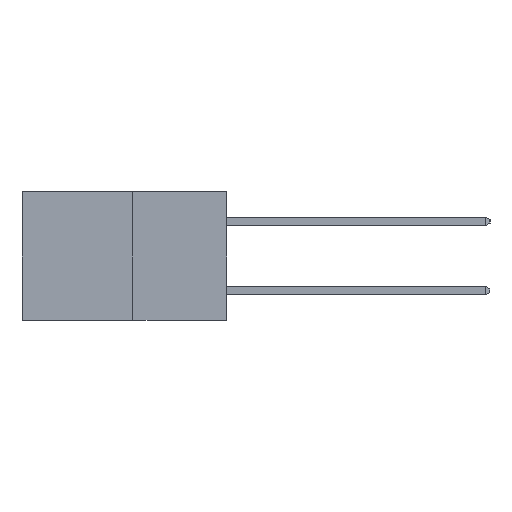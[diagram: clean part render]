
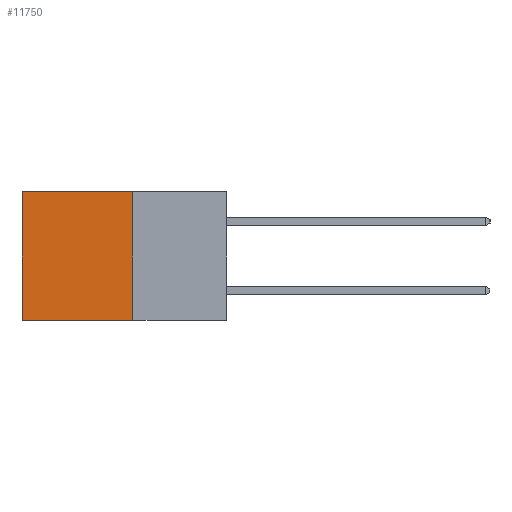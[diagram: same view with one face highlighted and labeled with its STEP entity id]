
A CAD part, left-side view. The second image highlights one B-rep face of the part: STEP entity #11750.
In plain terms, the highlighted planar face has unit normal (-1, 0, 0).
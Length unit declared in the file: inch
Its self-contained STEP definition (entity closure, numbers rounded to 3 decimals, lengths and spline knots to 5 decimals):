
#49 = ORIENTED_EDGE ( 'NONE', *, *, #5990, .T. ) ;
#1673 = LINE ( 'NONE', #11456, #5727 ) ;
#2010 = VERTEX_POINT ( 'NONE', #3660 ) ;
#2191 = DIRECTION ( 'NONE',  ( 0., 0., -1. ) ) ;
#3178 = EDGE_CURVE ( 'NONE', #15735, #7083, #20389, .T. ) ;
#3660 = CARTESIAN_POINT ( 'NONE',  ( 0.277, 0.27, 0. ) ) ;
#5144 = VECTOR ( 'NONE', #19757, 39.37008 ) ;
#5694 = LINE ( 'NONE', #19923, #5144 ) ;
#5727 = VECTOR ( 'NONE', #21216, 39.37008 ) ;
#5990 = EDGE_CURVE ( 'NONE', #2010, #15735, #5694, .T. ) ;
#6981 = ORIENTED_EDGE ( 'NONE', *, *, #3178, .T. ) ;
#6992 = CARTESIAN_POINT ( 'NONE',  ( 0.277, 0.27, -0.37 ) ) ;
#7083 = VERTEX_POINT ( 'NONE', #16394 ) ;
#7758 = FACE_OUTER_BOUND ( 'NONE', #13615, .T. ) ;
#8012 = ORIENTED_EDGE ( 'NONE', *, *, #16189, .F. ) ;
#10276 = DIRECTION ( 'NONE',  ( 0., 0., -1. ) ) ;
#11164 = VECTOR ( 'NONE', #2191, 39.37008 ) ;
#11213 = EDGE_CURVE ( 'NONE', #15390, #7083, #16667, .T. ) ;
#11267 = CARTESIAN_POINT ( 'NONE',  ( 0.277, 0.27, -0.37 ) ) ;
#11456 = CARTESIAN_POINT ( 'NONE',  ( 0.277, 0.27, -0.37 ) ) ;
#11750 = ADVANCED_FACE ( 'NONE', ( #7758 ), #11842, .F. ) ;
#11842 = PLANE ( 'NONE',  #14637 ) ;
#13615 = EDGE_LOOP ( 'NONE', ( #6981, #20023, #8012, #49 ) ) ;
#14637 = AXIS2_PLACEMENT_3D ( 'NONE', #6992, #20069, #10276 ) ;
#15370 = CARTESIAN_POINT ( 'NONE',  ( 0.277, 0.59, 0. ) ) ;
#15390 = VERTEX_POINT ( 'NONE', #11267 ) ;
#15735 = VERTEX_POINT ( 'NONE', #15370 ) ;
#16189 = EDGE_CURVE ( 'NONE', #2010, #15390, #1673, .T. ) ;
#16394 = CARTESIAN_POINT ( 'NONE',  ( 0.277, 0.59, -0.37 ) ) ;
#16667 = LINE ( 'NONE', #17223, #17208 ) ;
#17208 = VECTOR ( 'NONE', #20450, 39.37008 ) ;
#17223 = CARTESIAN_POINT ( 'NONE',  ( 0.277, 0.27, -0.37 ) ) ;
#17293 = CARTESIAN_POINT ( 'NONE',  ( 0.277, 0.59, -0.37 ) ) ;
#19757 = DIRECTION ( 'NONE',  ( 0., 1., 0. ) ) ;
#19923 = CARTESIAN_POINT ( 'NONE',  ( 0.277, 0.27, 0. ) ) ;
#20023 = ORIENTED_EDGE ( 'NONE', *, *, #11213, .F. ) ;
#20069 = DIRECTION ( 'NONE',  ( 1., 0., 0. ) ) ;
#20389 = LINE ( 'NONE', #17293, #11164 ) ;
#20450 = DIRECTION ( 'NONE',  ( 0., 1., 0. ) ) ;
#21216 = DIRECTION ( 'NONE',  ( 0., 0., -1. ) ) ;
